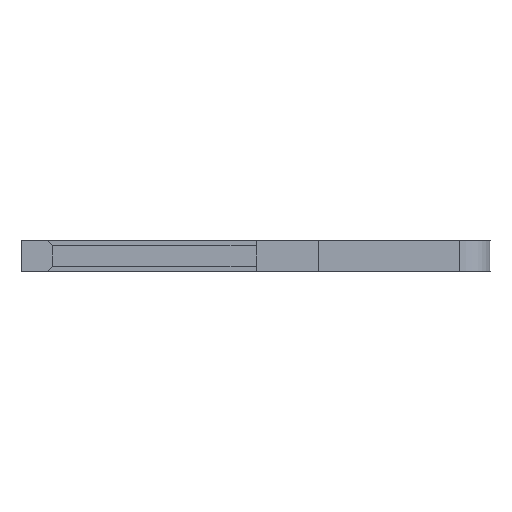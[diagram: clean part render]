
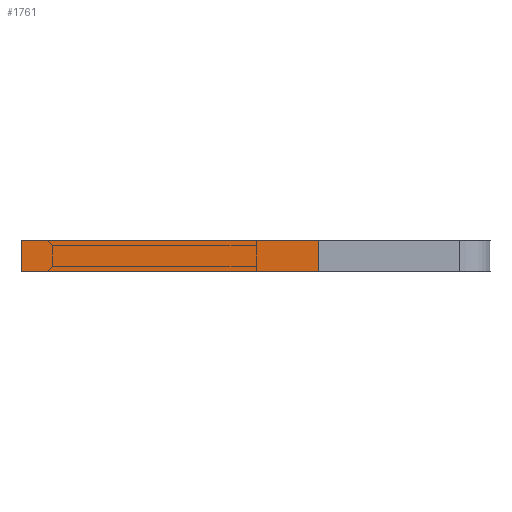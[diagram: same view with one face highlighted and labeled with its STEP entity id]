
A CAD part, left-side view. The second image highlights one B-rep face of the part: STEP entity #1761.
In plain terms, the highlighted face is planar.
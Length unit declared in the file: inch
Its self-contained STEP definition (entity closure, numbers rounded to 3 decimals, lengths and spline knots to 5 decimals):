
#5 = AXIS2_PLACEMENT_3D ( 'NONE', #2015, #1224, #209 ) ;
#30 = DIRECTION ( 'NONE',  ( -1., 0., 0. ) ) ;
#66 = VECTOR ( 'NONE', #664, 39.37008 ) ;
#209 = DIRECTION ( 'NONE',  ( 1., 0., 0. ) ) ;
#230 = DIRECTION ( 'NONE',  ( 0., 1., 0. ) ) ;
#414 = CARTESIAN_POINT ( 'NONE',  ( -0.01, 0.15, -0.04 ) ) ;
#416 = ORIENTED_EDGE ( 'NONE', *, *, #2049, .T. ) ;
#506 = VECTOR ( 'NONE', #30, 39.37008 ) ;
#658 = CARTESIAN_POINT ( 'NONE',  ( -0.01, 0.15, -0.04 ) ) ;
#664 = DIRECTION ( 'NONE',  ( 0., 1., 0. ) ) ;
#739 = ORIENTED_EDGE ( 'NONE', *, *, #2328, .F. ) ;
#809 = EDGE_CURVE ( 'NONE', #1638, #1935, #1963, .T. ) ;
#858 = ORIENTED_EDGE ( 'NONE', *, *, #1996, .T. ) ;
#1017 = CARTESIAN_POINT ( 'NONE',  ( 0.01, 0.15, -0.04 ) ) ;
#1048 = FACE_OUTER_BOUND ( 'NONE', #1836, .T. ) ;
#1224 = DIRECTION ( 'NONE',  ( 0., 0., 1. ) ) ;
#1265 = CARTESIAN_POINT ( 'NONE',  ( 0.01, -0.04, -0.04 ) ) ;
#1414 = VECTOR ( 'NONE', #2547, 39.37008 ) ;
#1575 = LINE ( 'NONE', #658, #1657 ) ;
#1638 = VERTEX_POINT ( 'NONE', #1017 ) ;
#1657 = VECTOR ( 'NONE', #230, 39.37008 ) ;
#1686 = LINE ( 'NONE', #1878, #66 ) ;
#1729 = CARTESIAN_POINT ( 'NONE',  ( 0.01, 0.15, -0.04 ) ) ;
#1761 = ADVANCED_FACE ( 'NONE', ( #1048 ), #1823, .F. ) ;
#1823 = PLANE ( 'NONE',  #5 ) ;
#1836 = EDGE_LOOP ( 'NONE', ( #858, #2356, #739, #416 ) ) ;
#1842 = CARTESIAN_POINT ( 'NONE',  ( -0.01, -0.04, -0.04 ) ) ;
#1878 = CARTESIAN_POINT ( 'NONE',  ( 0.01, 0.15, -0.04 ) ) ;
#1935 = VERTEX_POINT ( 'NONE', #414 ) ;
#1963 = LINE ( 'NONE', #1729, #1414 ) ;
#1996 = EDGE_CURVE ( 'NONE', #2322, #1935, #1575, .T. ) ;
#2015 = CARTESIAN_POINT ( 'NONE',  ( 0.01, 0.15, -0.04 ) ) ;
#2049 = EDGE_CURVE ( 'NONE', #2105, #2322, #2057, .T. ) ;
#2057 = LINE ( 'NONE', #1265, #506 ) ;
#2105 = VERTEX_POINT ( 'NONE', #2276 ) ;
#2276 = CARTESIAN_POINT ( 'NONE',  ( 0.01, -0.04, -0.04 ) ) ;
#2322 = VERTEX_POINT ( 'NONE', #1842 ) ;
#2328 = EDGE_CURVE ( 'NONE', #2105, #1638, #1686, .T. ) ;
#2356 = ORIENTED_EDGE ( 'NONE', *, *, #809, .F. ) ;
#2547 = DIRECTION ( 'NONE',  ( -1., 0., 0. ) ) ;
